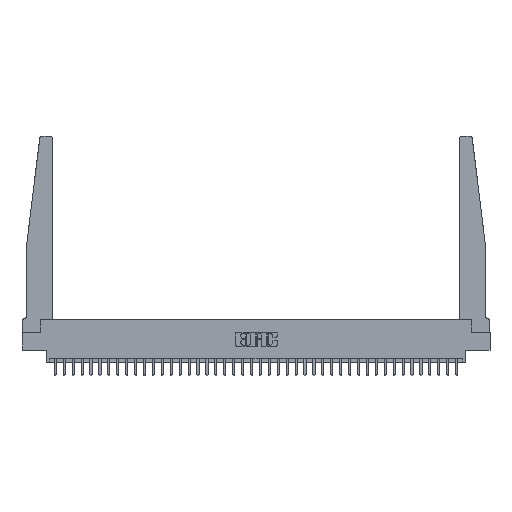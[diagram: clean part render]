
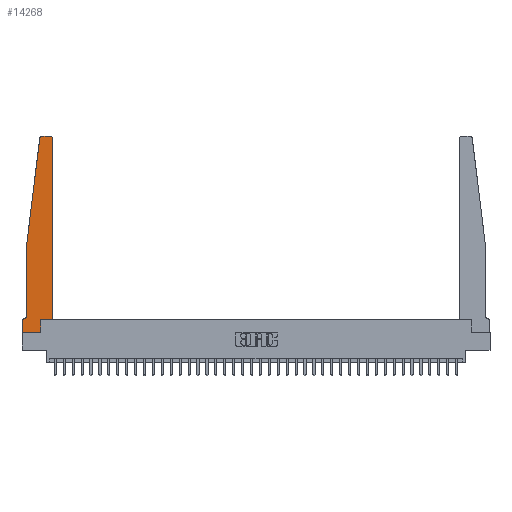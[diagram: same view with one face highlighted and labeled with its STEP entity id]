
A CAD part, top view. The second image highlights one B-rep face of the part: STEP entity #14268.
In plain terms, the highlighted planar face has unit normal (0, 0, 1).
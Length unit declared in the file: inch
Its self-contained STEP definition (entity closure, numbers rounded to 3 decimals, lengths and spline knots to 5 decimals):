
#6 = CIRCLE ( 'NONE', #2422, 0.03 ) ;
#74 = DIRECTION ( 'NONE',  ( 1., 0., 0. ) ) ;
#149 = EDGE_CURVE ( 'NONE', #801, #7153, #10457, .T. ) ;
#198 = DIRECTION ( 'NONE',  ( 0., 1., 0. ) ) ;
#209 = CARTESIAN_POINT ( 'NONE',  ( 0.065, 0.2375, 0.37 ) ) ;
#438 = ORIENTED_EDGE ( 'NONE', *, *, #24245, .T. ) ;
#801 = VERTEX_POINT ( 'NONE', #11964 ) ;
#984 = CARTESIAN_POINT ( 'NONE',  ( 0.2605, 0., 0.37 ) ) ;
#1239 = EDGE_CURVE ( 'NONE', #11168, #33245, #32602, .T. ) ;
#1623 = DIRECTION ( 'NONE',  ( 0., 0., 1. ) ) ;
#1629 = LINE ( 'NONE', #18201, #15333 ) ;
#1784 = DIRECTION ( 'NONE',  ( 0., 0., 1. ) ) ;
#1829 = FACE_OUTER_BOUND ( 'NONE', #22183, .T. ) ;
#1958 = ORIENTED_EDGE ( 'NONE', *, *, #8010, .T. ) ;
#2422 = AXIS2_PLACEMENT_3D ( 'NONE', #18015, #1623, #20695 ) ;
#2936 = ORIENTED_EDGE ( 'NONE', *, *, #3873, .T. ) ;
#3234 = VERTEX_POINT ( 'NONE', #23482 ) ;
#3432 = ORIENTED_EDGE ( 'NONE', *, *, #11122, .T. ) ;
#3650 = CIRCLE ( 'NONE', #11949, 0.03 ) ;
#3711 = CARTESIAN_POINT ( 'NONE',  ( 0.2605, 0.18, 0.37 ) ) ;
#3873 = EDGE_CURVE ( 'NONE', #6656, #11168, #3650, .T. ) ;
#4032 = EDGE_CURVE ( 'NONE', #3234, #4576, #5834, .T. ) ;
#4078 = ORIENTED_EDGE ( 'NONE', *, *, #4032, .T. ) ;
#4302 = CARTESIAN_POINT ( 'NONE',  ( 0.065, 0.1875, 0.37 ) ) ;
#4576 = VERTEX_POINT ( 'NONE', #31363 ) ;
#4729 = DIRECTION ( 'NONE',  ( 0., 1., 0. ) ) ;
#4973 = DIRECTION ( 'NONE',  ( 1., 0., 0. ) ) ;
#5187 = CARTESIAN_POINT ( 'NONE',  ( 0., 0., 0.37 ) ) ;
#5834 = LINE ( 'NONE', #5187, #19459 ) ;
#5908 = DIRECTION ( 'NONE',  ( 0., 0., -1. ) ) ;
#6336 = LINE ( 'NONE', #8378, #12746 ) ;
#6400 = DIRECTION ( 'NONE',  ( -1., 0., 0. ) ) ;
#6633 = CARTESIAN_POINT ( 'NONE',  ( 0.25, 2.75, 0.37 ) ) ;
#6656 = VERTEX_POINT ( 'NONE', #22842 ) ;
#7146 = ORIENTED_EDGE ( 'NONE', *, *, #23620, .T. ) ;
#7153 = VERTEX_POINT ( 'NONE', #30134 ) ;
#8010 = EDGE_CURVE ( 'NONE', #4576, #17215, #13794, .T. ) ;
#8378 = CARTESIAN_POINT ( 'NONE',  ( 0.2605, 0.18, 0.37 ) ) ;
#8946 = VERTEX_POINT ( 'NONE', #209 ) ;
#9831 = DIRECTION ( 'NONE',  ( -1., 0., 0. ) ) ;
#10457 = LINE ( 'NONE', #21495, #17697 ) ;
#10624 = EDGE_CURVE ( 'NONE', #33210, #3234, #23392, .T. ) ;
#11006 = PLANE ( 'NONE',  #20077 ) ;
#11122 = EDGE_CURVE ( 'NONE', #7153, #8946, #1629, .T. ) ;
#11168 = VERTEX_POINT ( 'NONE', #33974 ) ;
#11949 = AXIS2_PLACEMENT_3D ( 'NONE', #18171, #1784, #20874 ) ;
#11964 = CARTESIAN_POINT ( 'NONE',  ( 0.24675, 2.72367, 0.37 ) ) ;
#12746 = VECTOR ( 'NONE', #198, 39.37008 ) ;
#12755 = DIRECTION ( 'NONE',  ( 0., -1., 0. ) ) ;
#12872 = CARTESIAN_POINT ( 'NONE',  ( 0.425, 0.18, 0.37 ) ) ;
#13728 = CARTESIAN_POINT ( 'NONE',  ( 0., 0.1875, 0.37 ) ) ;
#13794 = LINE ( 'NONE', #21013, #33888 ) ;
#14162 = ORIENTED_EDGE ( 'NONE', *, *, #1239, .T. ) ;
#14268 = ADVANCED_FACE ( 'NONE', ( #1829 ), #11006, .T. ) ;
#14682 = ORIENTED_EDGE ( 'NONE', *, *, #19623, .T. ) ;
#15333 = VECTOR ( 'NONE', #12755, 39.37008 ) ;
#15371 = ORIENTED_EDGE ( 'NONE', *, *, #149, .T. ) ;
#15414 = AXIS2_PLACEMENT_3D ( 'NONE', #22162, #5908, #24816 ) ;
#16180 = CARTESIAN_POINT ( 'NONE',  ( 0.425, 0.18, 0.37 ) ) ;
#16472 = DIRECTION ( 'NONE',  ( 0., 0., 1. ) ) ;
#17038 = CIRCLE ( 'NONE', #15414, 0.05 ) ;
#17215 = VERTEX_POINT ( 'NONE', #984 ) ;
#17557 = EDGE_CURVE ( 'NONE', #33080, #24395, #21375, .T. ) ;
#17697 = VECTOR ( 'NONE', #21592, 39.37008 ) ;
#18015 = CARTESIAN_POINT ( 'NONE',  ( 0.27653, 2.72, 0.37 ) ) ;
#18053 = CARTESIAN_POINT ( 'NONE',  ( 0.27653, 2.75, 0.37 ) ) ;
#18171 = CARTESIAN_POINT ( 'NONE',  ( 0.395, 2.72, 0.37 ) ) ;
#18201 = CARTESIAN_POINT ( 'NONE',  ( 0.065, 1.25, 0.37 ) ) ;
#18553 = CARTESIAN_POINT ( 'NONE',  ( 0.425, 0.18, 0.37 ) ) ;
#19314 = ORIENTED_EDGE ( 'NONE', *, *, #30907, .T. ) ;
#19459 = VECTOR ( 'NONE', #26720, 39.37008 ) ;
#19623 = EDGE_CURVE ( 'NONE', #8946, #33210, #17038, .T. ) ;
#20077 = AXIS2_PLACEMENT_3D ( 'NONE', #13728, #16472, #74 ) ;
#20528 = VECTOR ( 'NONE', #4973, 39.37008 ) ;
#20695 = DIRECTION ( 'NONE',  ( 1., 0., 0. ) ) ;
#20874 = DIRECTION ( 'NONE',  ( 1., 0., 0. ) ) ;
#21013 = CARTESIAN_POINT ( 'NONE',  ( 0., 0., 0.37 ) ) ;
#21375 = LINE ( 'NONE', #18553, #20528 ) ;
#21495 = CARTESIAN_POINT ( 'NONE',  ( 0.065, 1.25, 0.37 ) ) ;
#21592 = DIRECTION ( 'NONE',  ( -0.122, -0.992, 0. ) ) ;
#22148 = VECTOR ( 'NONE', #4729, 39.37008 ) ;
#22162 = CARTESIAN_POINT ( 'NONE',  ( 0.015, 0.2375, 0.37 ) ) ;
#22183 = EDGE_LOOP ( 'NONE', ( #14162, #7146, #15371, #3432, #14682, #28193, #4078, #1958, #19314, #32084, #438, #2936 ) ) ;
#22555 = VECTOR ( 'NONE', #9831, 39.37008 ) ;
#22842 = CARTESIAN_POINT ( 'NONE',  ( 0.425, 2.72, 0.37 ) ) ;
#23392 = LINE ( 'NONE', #4302, #22555 ) ;
#23482 = CARTESIAN_POINT ( 'NONE',  ( 0., 0.1875, 0.37 ) ) ;
#23620 = EDGE_CURVE ( 'NONE', #33245, #801, #6, .T. ) ;
#23715 = DIRECTION ( 'NONE',  ( 1., 0., 0. ) ) ;
#24245 = EDGE_CURVE ( 'NONE', #24395, #6656, #29026, .T. ) ;
#24395 = VERTEX_POINT ( 'NONE', #16180 ) ;
#24816 = DIRECTION ( 'NONE',  ( -1., 0., 0. ) ) ;
#26720 = DIRECTION ( 'NONE',  ( 0., -1., 0. ) ) ;
#28193 = ORIENTED_EDGE ( 'NONE', *, *, #10624, .T. ) ;
#29026 = LINE ( 'NONE', #12872, #22148 ) ;
#30134 = CARTESIAN_POINT ( 'NONE',  ( 0.065, 1.25, 0.37 ) ) ;
#30907 = EDGE_CURVE ( 'NONE', #17215, #33080, #6336, .T. ) ;
#30948 = CARTESIAN_POINT ( 'NONE',  ( 0.015, 0.1875, 0.37 ) ) ;
#31363 = CARTESIAN_POINT ( 'NONE',  ( 0., 0., 0.37 ) ) ;
#31808 = VECTOR ( 'NONE', #6400, 39.37008 ) ;
#32084 = ORIENTED_EDGE ( 'NONE', *, *, #17557, .T. ) ;
#32602 = LINE ( 'NONE', #6633, #31808 ) ;
#33080 = VERTEX_POINT ( 'NONE', #3711 ) ;
#33210 = VERTEX_POINT ( 'NONE', #30948 ) ;
#33245 = VERTEX_POINT ( 'NONE', #18053 ) ;
#33888 = VECTOR ( 'NONE', #23715, 39.37008 ) ;
#33974 = CARTESIAN_POINT ( 'NONE',  ( 0.395, 2.75, 0.37 ) ) ;
